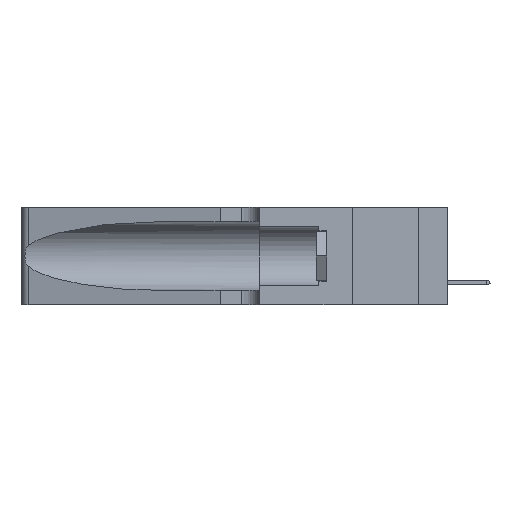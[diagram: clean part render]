
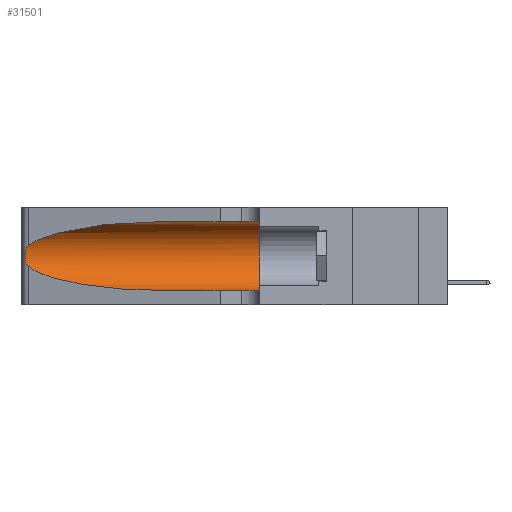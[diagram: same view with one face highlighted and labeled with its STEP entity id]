
A CAD part, left-side view. The second image highlights one B-rep face of the part: STEP entity #31501.
In plain terms, the highlighted cylindrical face has radius 3.308 mm (diameter 6.617 mm), a partial arc.
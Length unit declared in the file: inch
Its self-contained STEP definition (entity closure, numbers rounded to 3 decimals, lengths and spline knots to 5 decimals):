
#130 = CARTESIAN_POINT ( 'NONE',  ( 0.25487, 1.22718, 0.14631 ) ) ;
#596 = CIRCLE ( 'NONE', #31554, 0.13025 ) ;
#3824 = CARTESIAN_POINT ( 'NONE',  ( 0.25639, 1.23184, 0.21858 ) ) ;
#4047 = CARTESIAN_POINT ( 'NONE',  ( 0.18966, 0.96281, 0.05475 ) ) ;
#4348 = CARTESIAN_POINT ( 'NONE',  ( 0.25555, 1.22994, 0.2215 ) ) ;
#4995 = CARTESIAN_POINT ( 'NONE',  ( 0.26075, 1.23896, 0.178 ) ) ;
#5255 = VERTEX_POINT ( 'NONE', #7168 ) ;
#5306 = EDGE_CURVE ( 'NONE', #5255, #30656, #6253, .T. ) ;
#5756 = DIRECTION ( 'NONE',  ( 0., 1., 0. ) ) ;
#5955 = CARTESIAN_POINT ( 'NONE',  ( 0.2373, 1.15595, 0.08982 ) ) ;
#6253 = B_SPLINE_CURVE_WITH_KNOTS ( 'NONE', 3,
 ( #10089, #4348, #3824, #24233, #6762, #27147, #7803, #4995, #10855, #13319, #27797, #30940, #27924, #19152 ),
 .UNSPECIFIED., .F., .F.,
 ( 4, 2, 2, 2, 2, 2, 4 ),
 ( 0., 0.00027, 0.00053, 0.00107, 0.0016, 0.00187, 0.00214 ),
 .UNSPECIFIED. ) ;
#6463 = EDGE_CURVE ( 'NONE', #28426, #35498, #596, .T. ) ;
#6762 = CARTESIAN_POINT ( 'NONE',  ( 0.25854, 1.2359, 0.20912 ) ) ;
#6930 = VECTOR ( 'NONE', #11817, 39.37008 ) ;
#7049 = EDGE_CURVE ( 'NONE', #11939, #35498, #10117, .T. ) ;
#7168 = CARTESIAN_POINT ( 'NONE',  ( 0.25487, 1.22718, 0.22369 ) ) ;
#7203 = CARTESIAN_POINT ( 'NONE',  ( 0.1305, 0.35, 0.31525 ) ) ;
#7517 = EDGE_CURVE ( 'NONE', #30656, #11939, #34527, .T. ) ;
#7803 = CARTESIAN_POINT ( 'NONE',  ( 0.26075, 1.23896, 0.19203 ) ) ;
#9007 = ORIENTED_EDGE ( 'NONE', *, *, #7049, .T. ) ;
#9515 = DIRECTION ( 'NONE',  ( 0., 0., -1. ) ) ;
#10089 = CARTESIAN_POINT ( 'NONE',  ( 0.25487, 1.22718, 0.22369 ) ) ;
#10117 = LINE ( 'NONE', #29122, #6930 ) ;
#10855 = CARTESIAN_POINT ( 'NONE',  ( 0.26017, 1.23833, 0.17102 ) ) ;
#11395 = CYLINDRICAL_SURFACE ( 'NONE', #27041, 0.13025 ) ;
#11817 = DIRECTION ( 'NONE',  ( 0., -1., 0. ) ) ;
#11939 = VERTEX_POINT ( 'NONE', #33973 ) ;
#12654 = CARTESIAN_POINT ( 'NONE',  ( 0.1305, 0.72297, 0.31525 ) ) ;
#13319 = CARTESIAN_POINT ( 'NONE',  ( 0.25856, 1.23593, 0.16098 ) ) ;
#14036 = ORIENTED_EDGE ( 'NONE', *, *, #5306, .T. ) ;
#14361 = CARTESIAN_POINT ( 'NONE',  ( 0.1305, 0.35, 0.185 ) ) ;
#17316 = EDGE_CURVE ( 'NONE', #26261, #5255, #24518, .T. ) ;
#18724 = CARTESIAN_POINT ( 'NONE',  ( 0.1305, 1.61858, 0.31525 ) ) ;
#19152 = CARTESIAN_POINT ( 'NONE',  ( 0.25487, 1.22718, 0.14631 ) ) ;
#20151 = ORIENTED_EDGE ( 'NONE', *, *, #23998, .F. ) ;
#20758 = CARTESIAN_POINT ( 'NONE',  ( 0.1305, 0.35, 0.05475 ) ) ;
#21128 = CARTESIAN_POINT ( 'NONE',  ( 0.1305, 0.72297, 0.05475 ) ) ;
#21451 = ORIENTED_EDGE ( 'NONE', *, *, #17316, .T. ) ;
#22224 = CARTESIAN_POINT ( 'NONE',  ( 0.1305, 0.72297, 0.31525 ) ) ;
#22853 = CARTESIAN_POINT ( 'NONE',  ( 0.18966, 0.96281, 0.31525 ) ) ;
#23427 = CARTESIAN_POINT ( 'NONE',  ( 0.1305, 1.61858, 0.185 ) ) ;
#23998 = EDGE_CURVE ( 'NONE', #26261, #28426, #28201, .T. ) ;
#24233 = CARTESIAN_POINT ( 'NONE',  ( 0.25787, 1.23484, 0.2124 ) ) ;
#24273 = CARTESIAN_POINT ( 'NONE',  ( 0.25487, 1.22718, 0.14631 ) ) ;
#24518 =( BOUNDED_CURVE ( )  B_SPLINE_CURVE ( 3, ( #22224, #22853, #26246, #32305 ),
 .UNSPECIFIED., .F., .F. ) 
 B_SPLINE_CURVE_WITH_KNOTS ( ( 4, 4 ),
 ( 1.5708, 2.84003 ),
 .UNSPECIFIED. ) 
 CURVE ( )  GEOMETRIC_REPRESENTATION_ITEM ( )  RATIONAL_B_SPLINE_CURVE ( ( 1., 0.87, 0.87, 1. ) ) 
 REPRESENTATION_ITEM ( '' )  );
#24594 = ORIENTED_EDGE ( 'NONE', *, *, #6463, .F. ) ;
#26246 = CARTESIAN_POINT ( 'NONE',  ( 0.2373, 1.15595, 0.28018 ) ) ;
#26261 = VERTEX_POINT ( 'NONE', #12654 ) ;
#26420 = FACE_OUTER_BOUND ( 'NONE', #31013, .T. ) ;
#27041 = AXIS2_PLACEMENT_3D ( 'NONE', #23427, #34743, #9515 ) ;
#27147 = CARTESIAN_POINT ( 'NONE',  ( 0.26018, 1.23835, 0.19895 ) ) ;
#27797 = CARTESIAN_POINT ( 'NONE',  ( 0.25789, 1.23486, 0.15765 ) ) ;
#27924 = CARTESIAN_POINT ( 'NONE',  ( 0.25555, 1.22993, 0.14849 ) ) ;
#28201 = LINE ( 'NONE', #18724, #29075 ) ;
#28426 = VERTEX_POINT ( 'NONE', #7203 ) ;
#28945 = DIRECTION ( 'NONE',  ( 0., 0., 1. ) ) ;
#29075 = VECTOR ( 'NONE', #36254, 39.37008 ) ;
#29122 = CARTESIAN_POINT ( 'NONE',  ( 0.1305, 1.61858, 0.05475 ) ) ;
#29150 = ORIENTED_EDGE ( 'NONE', *, *, #7517, .T. ) ;
#30656 = VERTEX_POINT ( 'NONE', #24273 ) ;
#30940 = CARTESIAN_POINT ( 'NONE',  ( 0.25639, 1.23186, 0.15144 ) ) ;
#31013 = EDGE_LOOP ( 'NONE', ( #21451, #14036, #29150, #9007, #24594, #20151 ) ) ;
#31501 = ADVANCED_FACE ( 'NONE', ( #26420 ), #11395, .F. ) ;
#31554 = AXIS2_PLACEMENT_3D ( 'NONE', #14361, #5756, #28945 ) ;
#32305 = CARTESIAN_POINT ( 'NONE',  ( 0.25487, 1.22718, 0.22369 ) ) ;
#33973 = CARTESIAN_POINT ( 'NONE',  ( 0.1305, 0.72297, 0.05475 ) ) ;
#34527 =( BOUNDED_CURVE ( )  B_SPLINE_CURVE ( 3, ( #130, #5955, #4047, #21128 ),
 .UNSPECIFIED., .F., .F. ) 
 B_SPLINE_CURVE_WITH_KNOTS ( ( 4, 4 ),
 ( 3.44316, 4.71239 ),
 .UNSPECIFIED. ) 
 CURVE ( )  GEOMETRIC_REPRESENTATION_ITEM ( )  RATIONAL_B_SPLINE_CURVE ( ( 1., 0.87, 0.87, 1. ) ) 
 REPRESENTATION_ITEM ( '' )  );
#34743 = DIRECTION ( 'NONE',  ( 0., -1., 0. ) ) ;
#35498 = VERTEX_POINT ( 'NONE', #20758 ) ;
#36254 = DIRECTION ( 'NONE',  ( 0., -1., 0. ) ) ;
